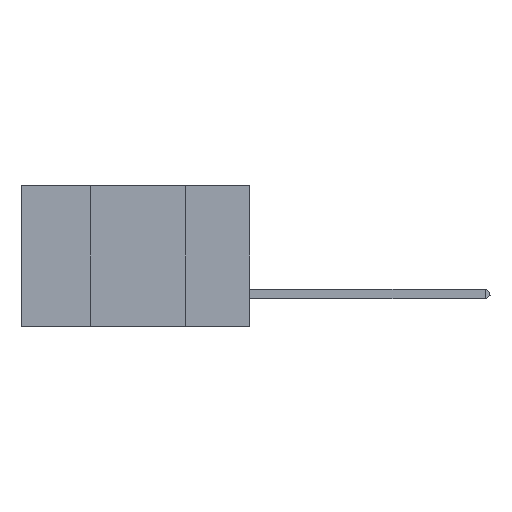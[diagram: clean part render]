
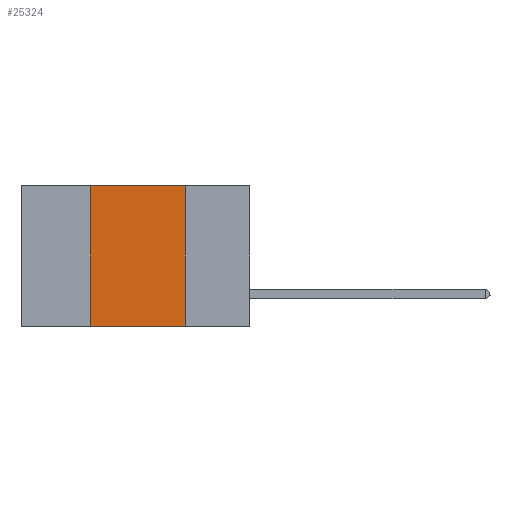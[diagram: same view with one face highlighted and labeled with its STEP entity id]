
A CAD part, left-side view. The second image highlights one B-rep face of the part: STEP entity #25324.
In plain terms, the highlighted planar face has unit normal (-1, 0, 0).
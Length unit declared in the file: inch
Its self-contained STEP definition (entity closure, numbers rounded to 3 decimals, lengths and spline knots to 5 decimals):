
#804 = CARTESIAN_POINT ( 'NONE',  ( 0., 0.6, 0. ) ) ;
#1627 = PLANE ( 'NONE',  #3094 ) ;
#1836 = CARTESIAN_POINT ( 'NONE',  ( 0., 0.6, 0. ) ) ;
#2675 = CARTESIAN_POINT ( 'NONE',  ( 0., 0.17, 0. ) ) ;
#3094 = AXIS2_PLACEMENT_3D ( 'NONE', #804, #24916, #47892 ) ;
#4351 = ORIENTED_EDGE ( 'NONE', *, *, #16529, .F. ) ;
#6445 = CARTESIAN_POINT ( 'NONE',  ( 0., 0.42, -0.37 ) ) ;
#8506 = VECTOR ( 'NONE', #31104, 39.37008 ) ;
#8832 = VECTOR ( 'NONE', #38027, 39.37008 ) ;
#10513 = VERTEX_POINT ( 'NONE', #21920 ) ;
#11213 = EDGE_CURVE ( 'NONE', #44547, #10513, #31940, .T. ) ;
#11233 = ORIENTED_EDGE ( 'NONE', *, *, #14817, .T. ) ;
#12942 = LINE ( 'NONE', #33411, #8832 ) ;
#13522 = CARTESIAN_POINT ( 'NONE',  ( 0., 0.42, 0. ) ) ;
#14817 = EDGE_CURVE ( 'NONE', #44547, #18389, #18616, .T. ) ;
#15835 = CARTESIAN_POINT ( 'NONE',  ( 0., 0.6, -0.37 ) ) ;
#16529 = EDGE_CURVE ( 'NONE', #10513, #31914, #21981, .T. ) ;
#16972 = EDGE_CURVE ( 'NONE', #31914, #18389, #12942, .T. ) ;
#18389 = VERTEX_POINT ( 'NONE', #32051 ) ;
#18616 = LINE ( 'NONE', #15835, #8506 ) ;
#19509 = VECTOR ( 'NONE', #47361, 39.37008 ) ;
#20612 = EDGE_LOOP ( 'NONE', ( #35752, #4351, #25261, #11233 ) ) ;
#21920 = CARTESIAN_POINT ( 'NONE',  ( 0., 0.42, 0. ) ) ;
#21981 = LINE ( 'NONE', #1836, #19509 ) ;
#24916 = DIRECTION ( 'NONE',  ( 1., 0., 0. ) ) ;
#25261 = ORIENTED_EDGE ( 'NONE', *, *, #11213, .F. ) ;
#25324 = ADVANCED_FACE ( 'NONE', ( #42501 ), #1627, .F. ) ;
#31104 = DIRECTION ( 'NONE',  ( 0., -1., 0. ) ) ;
#31914 = VERTEX_POINT ( 'NONE', #2675 ) ;
#31940 = LINE ( 'NONE', #13522, #39092 ) ;
#32051 = CARTESIAN_POINT ( 'NONE',  ( 0., 0.17, -0.37 ) ) ;
#33411 = CARTESIAN_POINT ( 'NONE',  ( 0., 0.17, 0. ) ) ;
#35752 = ORIENTED_EDGE ( 'NONE', *, *, #16972, .F. ) ;
#38027 = DIRECTION ( 'NONE',  ( 0., 0., -1. ) ) ;
#39092 = VECTOR ( 'NONE', #44044, 39.37008 ) ;
#42501 = FACE_OUTER_BOUND ( 'NONE', #20612, .T. ) ;
#44044 = DIRECTION ( 'NONE',  ( 0., 0., 1. ) ) ;
#44547 = VERTEX_POINT ( 'NONE', #6445 ) ;
#47361 = DIRECTION ( 'NONE',  ( 0., -1., 0. ) ) ;
#47892 = DIRECTION ( 'NONE',  ( 0., 0., -1. ) ) ;
